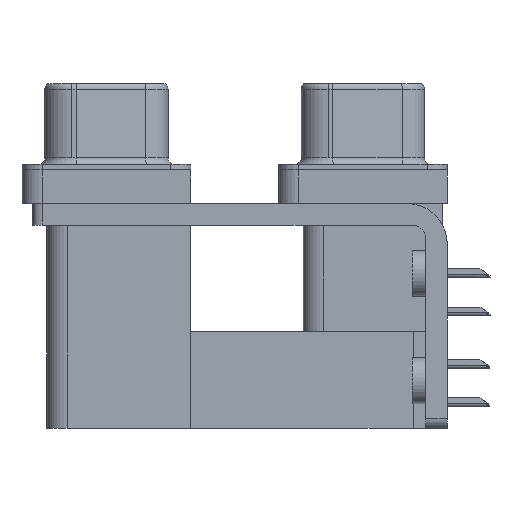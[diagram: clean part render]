
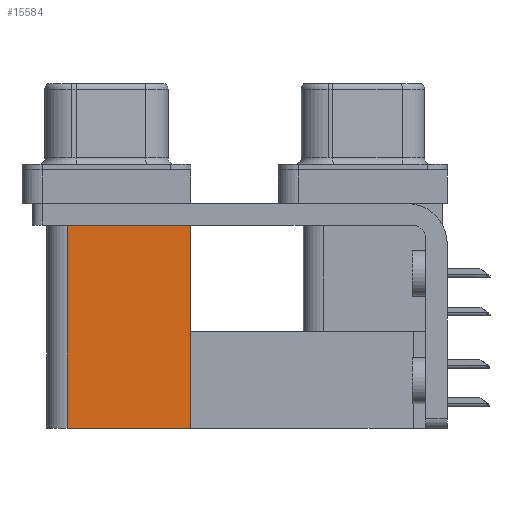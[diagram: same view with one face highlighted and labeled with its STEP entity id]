
A CAD part, left-side view. The second image highlights one B-rep face of the part: STEP entity #15584.
In plain terms, the highlighted planar face has unit normal (-1, 0, 0).
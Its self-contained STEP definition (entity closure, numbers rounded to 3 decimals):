
#555 = CARTESIAN_POINT ( 'NONE',  ( 3.765, 12.775, -2.5 ) ) ;
#1969 = DIRECTION ( 'NONE',  ( 0., 0., -1. ) ) ;
#2943 = LINE ( 'NONE', #21261, #30504 ) ;
#4369 = VERTEX_POINT ( 'NONE', #17775 ) ;
#4865 = LINE ( 'NONE', #12400, #9681 ) ;
#9681 = VECTOR ( 'NONE', #12757, 1000. ) ;
#11070 = CARTESIAN_POINT ( 'NONE',  ( 3.765, 12.775, -2.5 ) ) ;
#11625 = EDGE_CURVE ( 'NONE', #4369, #19129, #29832, .T. ) ;
#12400 = CARTESIAN_POINT ( 'NONE',  ( 3.765, 12.775, -19.2 ) ) ;
#12757 = DIRECTION ( 'NONE',  ( 0., 1., 0. ) ) ;
#14610 = CARTESIAN_POINT ( 'NONE',  ( 3.765, 12.775, -19.2 ) ) ;
#14820 = PLANE ( 'NONE',  #25838 ) ;
#14995 = FACE_OUTER_BOUND ( 'NONE', #15064, .T. ) ;
#15064 = EDGE_LOOP ( 'NONE', ( #32866, #16088, #17335, #33624 ) ) ;
#15584 = ADVANCED_FACE ( 'NONE', ( #14995 ), #14820, .F. ) ;
#16088 = ORIENTED_EDGE ( 'NONE', *, *, #24733, .F. ) ;
#17335 = ORIENTED_EDGE ( 'NONE', *, *, #23529, .F. ) ;
#17775 = CARTESIAN_POINT ( 'NONE',  ( 3.765, 12.775, -19.2 ) ) ;
#19129 = VERTEX_POINT ( 'NONE', #11070 ) ;
#19192 = DIRECTION ( 'NONE',  ( 0., 0., 1. ) ) ;
#19762 = CARTESIAN_POINT ( 'NONE',  ( 3.765, 21.975, -2.5 ) ) ;
#20718 = EDGE_CURVE ( 'NONE', #19129, #22414, #31503, .T. ) ;
#21261 = CARTESIAN_POINT ( 'NONE',  ( 3.765, 21.975, -19.2 ) ) ;
#22414 = VERTEX_POINT ( 'NONE', #19762 ) ;
#23032 = CARTESIAN_POINT ( 'NONE',  ( 3.765, 12.775, -19.2 ) ) ;
#23529 = EDGE_CURVE ( 'NONE', #4369, #29492, #4865, .T. ) ;
#23789 = VECTOR ( 'NONE', #28988, 1000. ) ;
#24733 = EDGE_CURVE ( 'NONE', #29492, #22414, #2943, .T. ) ;
#25438 = DIRECTION ( 'NONE',  ( 1., 0., 0. ) ) ;
#25838 = AXIS2_PLACEMENT_3D ( 'NONE', #23032, #25438, #1969 ) ;
#27271 = DIRECTION ( 'NONE',  ( 0., 0., 1. ) ) ;
#28988 = DIRECTION ( 'NONE',  ( 0., 1., 0. ) ) ;
#29492 = VERTEX_POINT ( 'NONE', #30910 ) ;
#29524 = VECTOR ( 'NONE', #27271, 1000. ) ;
#29832 = LINE ( 'NONE', #14610, #29524 ) ;
#30504 = VECTOR ( 'NONE', #19192, 1000. ) ;
#30910 = CARTESIAN_POINT ( 'NONE',  ( 3.765, 21.975, -19.2 ) ) ;
#31503 = LINE ( 'NONE', #555, #23789 ) ;
#32866 = ORIENTED_EDGE ( 'NONE', *, *, #20718, .T. ) ;
#33624 = ORIENTED_EDGE ( 'NONE', *, *, #11625, .T. ) ;
